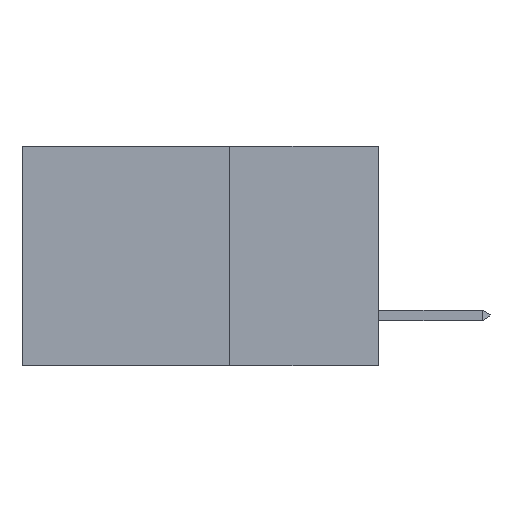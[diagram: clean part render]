
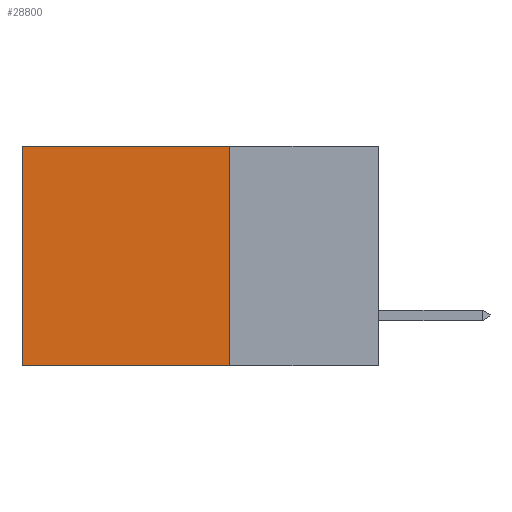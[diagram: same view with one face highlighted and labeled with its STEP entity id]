
A CAD part, left-side view. The second image highlights one B-rep face of the part: STEP entity #28800.
In plain terms, the highlighted planar face has unit normal (-1, 0, 0).
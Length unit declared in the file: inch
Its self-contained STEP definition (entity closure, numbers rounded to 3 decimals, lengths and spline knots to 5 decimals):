
#987 = CARTESIAN_POINT ( 'NONE',  ( 0.298, 0.25, 0. ) ) ;
#2010 = EDGE_CURVE ( 'NONE', #3309, #20586, #12577, .T. ) ;
#3309 = VERTEX_POINT ( 'NONE', #17788 ) ;
#4234 = VECTOR ( 'NONE', #6203, 39.37008 ) ;
#4349 = VECTOR ( 'NONE', #22860, 39.37008 ) ;
#6203 = DIRECTION ( 'NONE',  ( 0., 1., 0. ) ) ;
#6377 = EDGE_CURVE ( 'NONE', #17575, #19810, #12543, .T. ) ;
#6611 = DIRECTION ( 'NONE',  ( 1., 0., 0. ) ) ;
#6915 = VECTOR ( 'NONE', #28778, 39.37008 ) ;
#7422 = AXIS2_PLACEMENT_3D ( 'NONE', #17607, #6611, #8517 ) ;
#8086 = ORIENTED_EDGE ( 'NONE', *, *, #6377, .F. ) ;
#8239 = ORIENTED_EDGE ( 'NONE', *, *, #25092, .T. ) ;
#8334 = ORIENTED_EDGE ( 'NONE', *, *, #2010, .T. ) ;
#8517 = DIRECTION ( 'NONE',  ( 0., 0., -1. ) ) ;
#9110 = LINE ( 'NONE', #29245, #10517 ) ;
#10476 = FACE_OUTER_BOUND ( 'NONE', #17981, .T. ) ;
#10517 = VECTOR ( 'NONE', #18674, 39.37008 ) ;
#11082 = PLANE ( 'NONE',  #7422 ) ;
#12519 = EDGE_CURVE ( 'NONE', #19810, #20586, #13810, .T. ) ;
#12543 = LINE ( 'NONE', #29200, #4349 ) ;
#12577 = LINE ( 'NONE', #14767, #6915 ) ;
#13810 = LINE ( 'NONE', #20070, #4234 ) ;
#14767 = CARTESIAN_POINT ( 'NONE',  ( 0.298, 0.6, 0. ) ) ;
#15248 = CARTESIAN_POINT ( 'NONE',  ( 0.298, 0.6, -0.37 ) ) ;
#17575 = VERTEX_POINT ( 'NONE', #987 ) ;
#17607 = CARTESIAN_POINT ( 'NONE',  ( 0.298, 0.25, 0. ) ) ;
#17788 = CARTESIAN_POINT ( 'NONE',  ( 0.298, 0.6, 0. ) ) ;
#17981 = EDGE_LOOP ( 'NONE', ( #8334, #26035, #8086, #8239 ) ) ;
#18385 = CARTESIAN_POINT ( 'NONE',  ( 0.298, 0.25, -0.37 ) ) ;
#18674 = DIRECTION ( 'NONE',  ( 0., 1., 0. ) ) ;
#19810 = VERTEX_POINT ( 'NONE', #18385 ) ;
#20070 = CARTESIAN_POINT ( 'NONE',  ( 0.298, 0.25, -0.37 ) ) ;
#20586 = VERTEX_POINT ( 'NONE', #15248 ) ;
#22860 = DIRECTION ( 'NONE',  ( 0., 0., -1. ) ) ;
#25092 = EDGE_CURVE ( 'NONE', #17575, #3309, #9110, .T. ) ;
#26035 = ORIENTED_EDGE ( 'NONE', *, *, #12519, .F. ) ;
#28778 = DIRECTION ( 'NONE',  ( 0., 0., -1. ) ) ;
#28800 = ADVANCED_FACE ( 'NONE', ( #10476 ), #11082, .F. ) ;
#29200 = CARTESIAN_POINT ( 'NONE',  ( 0.298, 0.25, 0. ) ) ;
#29245 = CARTESIAN_POINT ( 'NONE',  ( 0.298, 0.25, 0. ) ) ;
